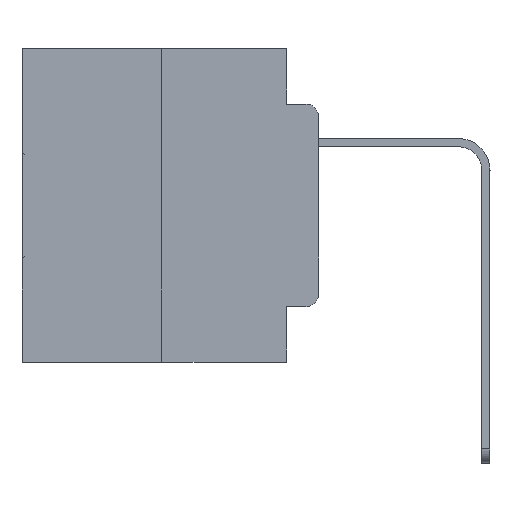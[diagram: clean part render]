
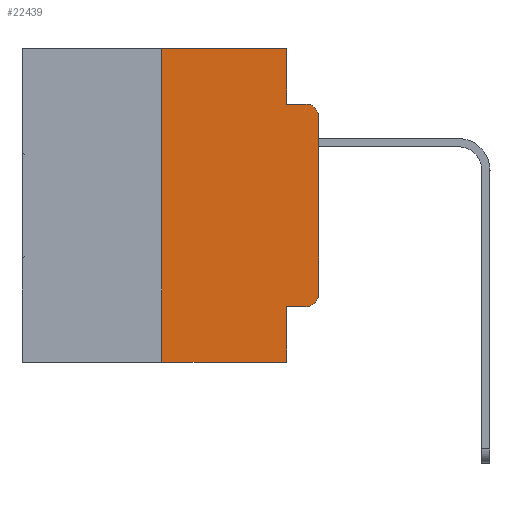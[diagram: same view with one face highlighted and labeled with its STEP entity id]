
A CAD part, left-side view. The second image highlights one B-rep face of the part: STEP entity #22439.
In plain terms, the highlighted planar face has unit normal (-1, 0, 0).
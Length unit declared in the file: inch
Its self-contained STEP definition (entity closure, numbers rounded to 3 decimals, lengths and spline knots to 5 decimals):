
#46 = EDGE_CURVE ( 'NONE', #14865, #6352, #25723, .T. ) ;
#395 = ORIENTED_EDGE ( 'NONE', *, *, #8111, .T. ) ;
#731 = DIRECTION ( 'NONE',  ( -1., 0., 0. ) ) ;
#1216 = CARTESIAN_POINT ( 'NONE',  ( 0., 0.02, -0.4115 ) ) ;
#1223 = CARTESIAN_POINT ( 'NONE',  ( 0., 0.02, -0.0885 ) ) ;
#1295 = CARTESIAN_POINT ( 'NONE',  ( 0., 0.051, -0.0885 ) ) ;
#1555 = CARTESIAN_POINT ( 'NONE',  ( 0., 0.473, 0. ) ) ;
#1556 = EDGE_LOOP ( 'NONE', ( #25649, #395, #14088, #3105, #4318, #2968, #18254, #25182, #19612, #18026 ) ) ;
#2255 = DIRECTION ( 'NONE',  ( 0., 0., 1. ) ) ;
#2479 = VERTEX_POINT ( 'NONE', #14950 ) ;
#2968 = ORIENTED_EDGE ( 'NONE', *, *, #20710, .F. ) ;
#3095 = CARTESIAN_POINT ( 'NONE',  ( 0., 0.051, 0. ) ) ;
#3105 = ORIENTED_EDGE ( 'NONE', *, *, #10543, .F. ) ;
#3179 = VERTEX_POINT ( 'NONE', #9693 ) ;
#3383 = CARTESIAN_POINT ( 'NONE',  ( 0., 0., -0.1085 ) ) ;
#3445 = AXIS2_PLACEMENT_3D ( 'NONE', #20559, #731, #18880 ) ;
#4129 = VECTOR ( 'NONE', #2255, 39.37008 ) ;
#4271 = CARTESIAN_POINT ( 'NONE',  ( 0., 0.051, 0. ) ) ;
#4318 = ORIENTED_EDGE ( 'NONE', *, *, #46, .F. ) ;
#4568 = CARTESIAN_POINT ( 'NONE',  ( 0., 0.25, 0. ) ) ;
#4794 = CARTESIAN_POINT ( 'NONE',  ( 0., 0., 0. ) ) ;
#5292 = VECTOR ( 'NONE', #11967, 39.37008 ) ;
#5673 = CARTESIAN_POINT ( 'NONE',  ( 0., 0.051, -0.4115 ) ) ;
#6352 = VERTEX_POINT ( 'NONE', #8217 ) ;
#6460 = VERTEX_POINT ( 'NONE', #15193 ) ;
#6515 = DIRECTION ( 'NONE',  ( 0., 0., -1. ) ) ;
#6536 = EDGE_CURVE ( 'NONE', #6460, #20062, #20484, .T. ) ;
#6926 = DIRECTION ( 'NONE',  ( 0., 0., 1. ) ) ;
#7117 = VERTEX_POINT ( 'NONE', #10898 ) ;
#8111 = EDGE_CURVE ( 'NONE', #20062, #12941, #20032, .T. ) ;
#8202 = EDGE_CURVE ( 'NONE', #7117, #12941, #17938, .T. ) ;
#8217 = CARTESIAN_POINT ( 'NONE',  ( 0., 0.051, 0. ) ) ;
#8376 = DIRECTION ( 'NONE',  ( 0., 0., -1. ) ) ;
#9693 = CARTESIAN_POINT ( 'NONE',  ( 0., 0.051, -0.4115 ) ) ;
#10178 = VECTOR ( 'NONE', #21039, 39.37008 ) ;
#10543 = EDGE_CURVE ( 'NONE', #6352, #7117, #14310, .T. ) ;
#10593 = DIRECTION ( 'NONE',  ( 0., -1., 0. ) ) ;
#10898 = CARTESIAN_POINT ( 'NONE',  ( 0., 0.051, -0.0885 ) ) ;
#11346 = VECTOR ( 'NONE', #16837, 39.37008 ) ;
#11967 = DIRECTION ( 'NONE',  ( 0., 0., -1. ) ) ;
#12941 = VERTEX_POINT ( 'NONE', #1223 ) ;
#13132 = LINE ( 'NONE', #4271, #16959 ) ;
#13490 = CIRCLE ( 'NONE', #3445, 0.02 ) ;
#13538 = EDGE_CURVE ( 'NONE', #15057, #6460, #13490, .T. ) ;
#13702 = VECTOR ( 'NONE', #10593, 39.37008 ) ;
#14088 = ORIENTED_EDGE ( 'NONE', *, *, #8202, .F. ) ;
#14246 = CARTESIAN_POINT ( 'NONE',  ( 0., 0.25, -0.5 ) ) ;
#14310 = LINE ( 'NONE', #3095, #5292 ) ;
#14760 = VERTEX_POINT ( 'NONE', #14246 ) ;
#14801 = CARTESIAN_POINT ( 'NONE',  ( 0., 0.02, -0.1085 ) ) ;
#14865 = VERTEX_POINT ( 'NONE', #16487 ) ;
#14950 = CARTESIAN_POINT ( 'NONE',  ( 0., 0.051, -0.5 ) ) ;
#14971 = CARTESIAN_POINT ( 'NONE',  ( 0., 0.473, 0. ) ) ;
#15057 = VERTEX_POINT ( 'NONE', #1216 ) ;
#15061 = DIRECTION ( 'NONE',  ( 1., 0., 0. ) ) ;
#15193 = CARTESIAN_POINT ( 'NONE',  ( 0., 0., -0.3915 ) ) ;
#15234 = CARTESIAN_POINT ( 'NONE',  ( 0., 0.473, -0.5 ) ) ;
#16079 = LINE ( 'NONE', #5673, #10178 ) ;
#16487 = CARTESIAN_POINT ( 'NONE',  ( 0., 0.25, 0. ) ) ;
#16494 = EDGE_CURVE ( 'NONE', #14760, #2479, #19598, .T. ) ;
#16837 = DIRECTION ( 'NONE',  ( 0., -1., 0. ) ) ;
#16959 = VECTOR ( 'NONE', #6515, 39.37008 ) ;
#17402 = EDGE_CURVE ( 'NONE', #3179, #15057, #16079, .T. ) ;
#17938 = LINE ( 'NONE', #1295, #11346 ) ;
#18026 = ORIENTED_EDGE ( 'NONE', *, *, #13538, .T. ) ;
#18254 = ORIENTED_EDGE ( 'NONE', *, *, #16494, .T. ) ;
#18880 = DIRECTION ( 'NONE',  ( 0., 0., -1. ) ) ;
#19001 = VECTOR ( 'NONE', #6926, 39.37008 ) ;
#19064 = DIRECTION ( 'NONE',  ( 0., 0., -1. ) ) ;
#19598 = LINE ( 'NONE', #15234, #13702 ) ;
#19612 = ORIENTED_EDGE ( 'NONE', *, *, #17402, .T. ) ;
#19786 = EDGE_CURVE ( 'NONE', #3179, #2479, #13132, .T. ) ;
#20032 = CIRCLE ( 'NONE', #25330, 0.02 ) ;
#20062 = VERTEX_POINT ( 'NONE', #3383 ) ;
#20417 = LINE ( 'NONE', #4568, #19001 ) ;
#20476 = DIRECTION ( 'NONE',  ( 0., -1., 0. ) ) ;
#20484 = LINE ( 'NONE', #4794, #4129 ) ;
#20559 = CARTESIAN_POINT ( 'NONE',  ( 0., 0.02, -0.3915 ) ) ;
#20710 = EDGE_CURVE ( 'NONE', #14760, #14865, #20417, .T. ) ;
#21039 = DIRECTION ( 'NONE',  ( 0., -1., 0. ) ) ;
#21867 = VECTOR ( 'NONE', #20476, 39.37008 ) ;
#22072 = FACE_OUTER_BOUND ( 'NONE', #1556, .T. ) ;
#22439 = ADVANCED_FACE ( 'NONE', ( #22072 ), #26050, .F. ) ;
#24184 = AXIS2_PLACEMENT_3D ( 'NONE', #1555, #15061, #8376 ) ;
#25182 = ORIENTED_EDGE ( 'NONE', *, *, #19786, .F. ) ;
#25330 = AXIS2_PLACEMENT_3D ( 'NONE', #14801, #25988, #19064 ) ;
#25649 = ORIENTED_EDGE ( 'NONE', *, *, #6536, .T. ) ;
#25723 = LINE ( 'NONE', #14971, #21867 ) ;
#25988 = DIRECTION ( 'NONE',  ( -1., 0., 0. ) ) ;
#26050 = PLANE ( 'NONE',  #24184 ) ;
